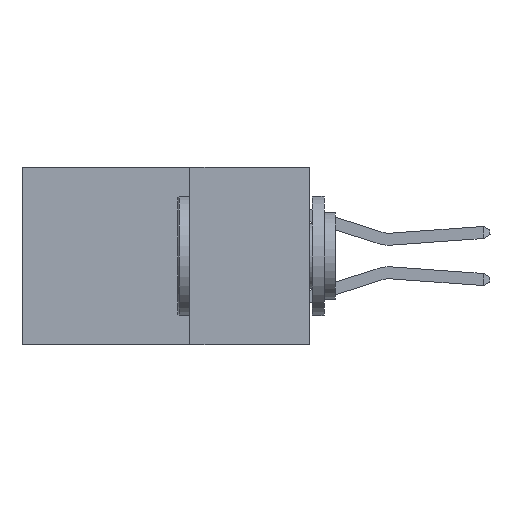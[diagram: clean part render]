
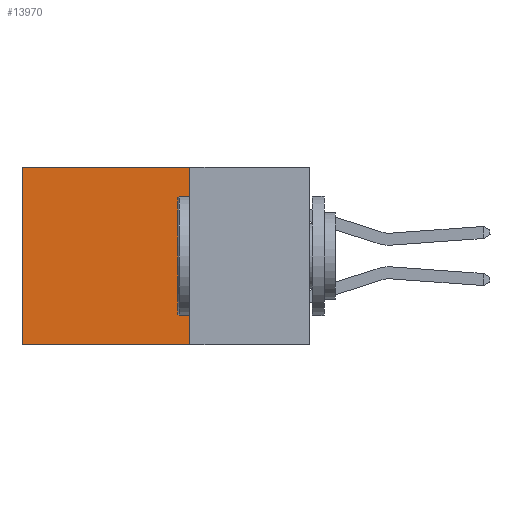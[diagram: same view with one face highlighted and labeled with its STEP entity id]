
A CAD part, left-side view. The second image highlights one B-rep face of the part: STEP entity #13970.
In plain terms, the highlighted planar face has unit normal (-1, 0, 0).
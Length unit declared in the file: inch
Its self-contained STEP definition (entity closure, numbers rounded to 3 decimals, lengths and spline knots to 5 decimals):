
#99 = EDGE_CURVE ( 'NONE', #8376, #11860, #14992, .T. ) ;
#284 = VERTEX_POINT ( 'NONE', #5218 ) ;
#605 = EDGE_LOOP ( 'NONE', ( #7558, #9041, #11488, #2339 ) ) ;
#647 = VECTOR ( 'NONE', #13157, 39.37008 ) ;
#1441 = CARTESIAN_POINT ( 'NONE',  ( 0.2615, 0.6, -0.37 ) ) ;
#2339 = ORIENTED_EDGE ( 'NONE', *, *, #99, .T. ) ;
#2431 = VERTEX_POINT ( 'NONE', #1441 ) ;
#3759 = CARTESIAN_POINT ( 'NONE',  ( 0.2615, 0.6, 0. ) ) ;
#3773 = EDGE_CURVE ( 'NONE', #11860, #2431, #10039, .T. ) ;
#4793 = EDGE_CURVE ( 'NONE', #284, #2431, #11371, .T. ) ;
#4919 = CARTESIAN_POINT ( 'NONE',  ( 0.2615, 0.6, -0.37 ) ) ;
#5218 = CARTESIAN_POINT ( 'NONE',  ( 0.2615, 0.25, -0.37 ) ) ;
#5444 = CARTESIAN_POINT ( 'NONE',  ( 0.2615, 0.25, -0.37 ) ) ;
#5517 = DIRECTION ( 'NONE',  ( 0., 0., -1. ) ) ;
#6013 = CARTESIAN_POINT ( 'NONE',  ( 0.2615, 0.25, -0.37 ) ) ;
#6792 = CARTESIAN_POINT ( 'NONE',  ( 0.2615, 0.25, -0.37 ) ) ;
#7088 = EDGE_CURVE ( 'NONE', #8376, #284, #14115, .T. ) ;
#7558 = ORIENTED_EDGE ( 'NONE', *, *, #3773, .T. ) ;
#8376 = VERTEX_POINT ( 'NONE', #12684 ) ;
#8860 = DIRECTION ( 'NONE',  ( 0., 1., 0. ) ) ;
#9041 = ORIENTED_EDGE ( 'NONE', *, *, #4793, .F. ) ;
#9120 = AXIS2_PLACEMENT_3D ( 'NONE', #6792, #15376, #5517 ) ;
#9176 = DIRECTION ( 'NONE',  ( 0., 1., 0. ) ) ;
#9333 = FACE_OUTER_BOUND ( 'NONE', #605, .T. ) ;
#10039 = LINE ( 'NONE', #4919, #14889 ) ;
#11087 = DIRECTION ( 'NONE',  ( 0., 0., -1. ) ) ;
#11371 = LINE ( 'NONE', #5444, #11539 ) ;
#11381 = CARTESIAN_POINT ( 'NONE',  ( 0.2615, 0.25, 0. ) ) ;
#11488 = ORIENTED_EDGE ( 'NONE', *, *, #7088, .F. ) ;
#11539 = VECTOR ( 'NONE', #9176, 39.37008 ) ;
#11562 = VECTOR ( 'NONE', #8860, 39.37008 ) ;
#11860 = VERTEX_POINT ( 'NONE', #3759 ) ;
#12684 = CARTESIAN_POINT ( 'NONE',  ( 0.2615, 0.25, 0. ) ) ;
#12732 = PLANE ( 'NONE',  #9120 ) ;
#13157 = DIRECTION ( 'NONE',  ( 0., 0., -1. ) ) ;
#13970 = ADVANCED_FACE ( 'NONE', ( #9333 ), #12732, .F. ) ;
#14115 = LINE ( 'NONE', #6013, #647 ) ;
#14889 = VECTOR ( 'NONE', #11087, 39.37008 ) ;
#14992 = LINE ( 'NONE', #11381, #11562 ) ;
#15376 = DIRECTION ( 'NONE',  ( 1., 0., 0. ) ) ;
